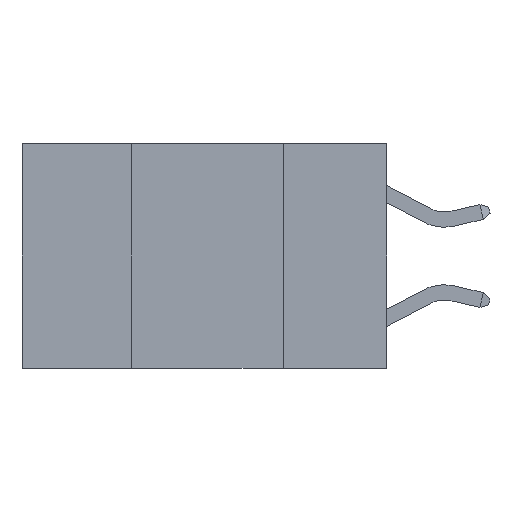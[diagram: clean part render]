
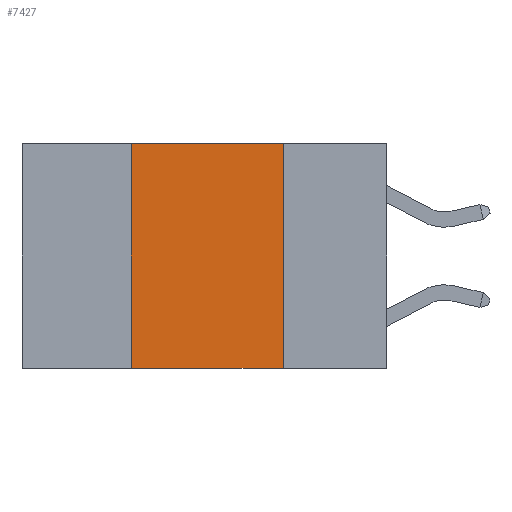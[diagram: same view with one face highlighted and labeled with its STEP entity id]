
A CAD part, left-side view. The second image highlights one B-rep face of the part: STEP entity #7427.
In plain terms, the highlighted planar face has unit normal (-1, 0, 0).
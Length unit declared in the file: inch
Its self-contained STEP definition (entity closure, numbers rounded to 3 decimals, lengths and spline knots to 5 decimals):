
#285 = ORIENTED_EDGE ( 'NONE', *, *, #6825, .F. ) ;
#852 = VERTEX_POINT ( 'NONE', #6367 ) ;
#2564 = LINE ( 'NONE', #4761, #12217 ) ;
#3277 = DIRECTION ( 'NONE',  ( 0., 0., -1. ) ) ;
#3351 = VECTOR ( 'NONE', #18395, 39.37008 ) ;
#3680 = VECTOR ( 'NONE', #3277, 39.37008 ) ;
#3699 = VERTEX_POINT ( 'NONE', #10674 ) ;
#3824 = VERTEX_POINT ( 'NONE', #15039 ) ;
#4130 = LINE ( 'NONE', #13325, #3680 ) ;
#4248 = FACE_OUTER_BOUND ( 'NONE', #8992, .T. ) ;
#4458 = DIRECTION ( 'NONE',  ( 1., 0., 0. ) ) ;
#4735 = ORIENTED_EDGE ( 'NONE', *, *, #6324, .T. ) ;
#4761 = CARTESIAN_POINT ( 'NONE',  ( 0., 0.6, -0.37 ) ) ;
#5156 = ORIENTED_EDGE ( 'NONE', *, *, #17340, .F. ) ;
#5926 = ORIENTED_EDGE ( 'NONE', *, *, #14549, .F. ) ;
#6324 = EDGE_CURVE ( 'NONE', #3699, #14573, #2564, .T. ) ;
#6367 = CARTESIAN_POINT ( 'NONE',  ( 0., 0.17, 0. ) ) ;
#6825 = EDGE_CURVE ( 'NONE', #3699, #3824, #17850, .T. ) ;
#7427 = ADVANCED_FACE ( 'NONE', ( #4248 ), #13087, .F. ) ;
#8992 = EDGE_LOOP ( 'NONE', ( #5156, #5926, #285, #4735 ) ) ;
#10674 = CARTESIAN_POINT ( 'NONE',  ( 0., 0.42, -0.37 ) ) ;
#11466 = CARTESIAN_POINT ( 'NONE',  ( 0., 0.6, 0. ) ) ;
#11492 = LINE ( 'NONE', #11466, #3351 ) ;
#11625 = CARTESIAN_POINT ( 'NONE',  ( 0., 0.6, 0. ) ) ;
#11755 = CARTESIAN_POINT ( 'NONE',  ( 0., 0.42, 0. ) ) ;
#12013 = DIRECTION ( 'NONE',  ( 0., -1., 0. ) ) ;
#12217 = VECTOR ( 'NONE', #12013, 39.37008 ) ;
#13087 = PLANE ( 'NONE',  #15271 ) ;
#13176 = DIRECTION ( 'NONE',  ( 0., 0., 1. ) ) ;
#13325 = CARTESIAN_POINT ( 'NONE',  ( 0., 0.17, 0. ) ) ;
#14129 = VECTOR ( 'NONE', #13176, 39.37008 ) ;
#14454 = DIRECTION ( 'NONE',  ( 0., 0., -1. ) ) ;
#14549 = EDGE_CURVE ( 'NONE', #3824, #852, #11492, .T. ) ;
#14573 = VERTEX_POINT ( 'NONE', #18448 ) ;
#15039 = CARTESIAN_POINT ( 'NONE',  ( 0., 0.42, 0. ) ) ;
#15271 = AXIS2_PLACEMENT_3D ( 'NONE', #11625, #4458, #14454 ) ;
#17340 = EDGE_CURVE ( 'NONE', #852, #14573, #4130, .T. ) ;
#17850 = LINE ( 'NONE', #11755, #14129 ) ;
#18395 = DIRECTION ( 'NONE',  ( 0., -1., 0. ) ) ;
#18448 = CARTESIAN_POINT ( 'NONE',  ( 0., 0.17, -0.37 ) ) ;
